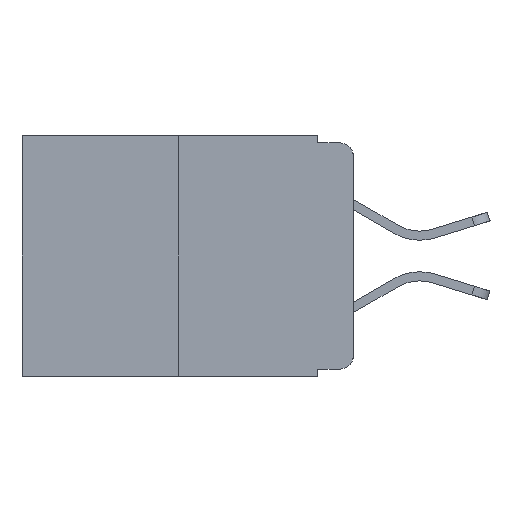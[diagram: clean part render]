
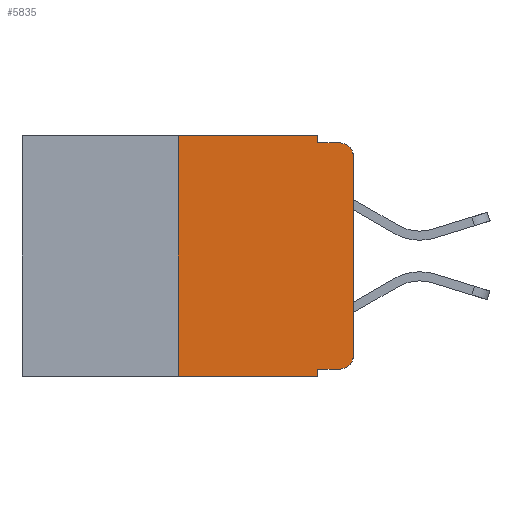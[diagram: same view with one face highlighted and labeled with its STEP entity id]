
A CAD part, left-side view. The second image highlights one B-rep face of the part: STEP entity #5835.
In plain terms, the highlighted planar face has unit normal (-1, 0, 0).
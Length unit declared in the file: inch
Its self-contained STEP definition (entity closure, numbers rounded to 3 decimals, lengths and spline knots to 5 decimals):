
#280 = DIRECTION ( 'NONE',  ( 0., 0., 1. ) ) ;
#578 = ORIENTED_EDGE ( 'NONE', *, *, #2444, .T. ) ;
#847 = DIRECTION ( 'NONE',  ( 0., 0., 1. ) ) ;
#1234 = CARTESIAN_POINT ( 'NONE',  ( 0., 0.25, 0. ) ) ;
#1261 = DIRECTION ( 'NONE',  ( 0., 0., -1. ) ) ;
#1451 = CARTESIAN_POINT ( 'NONE',  ( 0., 0., 0. ) ) ;
#1486 = DIRECTION ( 'NONE',  ( -1., 0., 0. ) ) ;
#1770 = EDGE_CURVE ( 'NONE', #8719, #7977, #2760, .T. ) ;
#1995 = VERTEX_POINT ( 'NONE', #3878 ) ;
#2293 = ORIENTED_EDGE ( 'NONE', *, *, #6491, .T. ) ;
#2437 = AXIS2_PLACEMENT_3D ( 'NONE', #7546, #1486, #8448 ) ;
#2444 = EDGE_CURVE ( 'NONE', #3549, #8719, #9752, .T. ) ;
#2611 = VECTOR ( 'NONE', #847, 39.37008 ) ;
#2659 = AXIS2_PLACEMENT_3D ( 'NONE', #9032, #11197, #12497 ) ;
#2755 = AXIS2_PLACEMENT_3D ( 'NONE', #6272, #4415, #4401 ) ;
#2760 = CIRCLE ( 'NONE', #2659, 0.02 ) ;
#2763 = CARTESIAN_POINT ( 'NONE',  ( 0., 0.473, 0. ) ) ;
#3030 = EDGE_LOOP ( 'NONE', ( #9432, #2293, #4907, #12263, #5556, #6881, #4759, #7770, #578, #8630 ) ) ;
#3115 = EDGE_CURVE ( 'NONE', #3549, #4345, #4777, .T. ) ;
#3549 = VERTEX_POINT ( 'NONE', #8162 ) ;
#3554 = VECTOR ( 'NONE', #8845, 39.37008 ) ;
#3674 = CARTESIAN_POINT ( 'NONE',  ( 0., 0., -0.313 ) ) ;
#3776 = EDGE_CURVE ( 'NONE', #5357, #1995, #7906, .T. ) ;
#3878 = CARTESIAN_POINT ( 'NONE',  ( 0., 0.25, 0. ) ) ;
#4345 = VERTEX_POINT ( 'NONE', #9505 ) ;
#4401 = DIRECTION ( 'NONE',  ( 0., 0., -1. ) ) ;
#4415 = DIRECTION ( 'NONE',  ( 1., 0., 0. ) ) ;
#4565 = DIRECTION ( 'NONE',  ( 0., -1., 0. ) ) ;
#4583 = CARTESIAN_POINT ( 'NONE',  ( 0., 0.051, -0.01 ) ) ;
#4759 = ORIENTED_EDGE ( 'NONE', *, *, #12245, .T. ) ;
#4777 = LINE ( 'NONE', #7247, #9591 ) ;
#4907 = ORIENTED_EDGE ( 'NONE', *, *, #5789, .F. ) ;
#5076 = EDGE_CURVE ( 'NONE', #10457, #11267, #9008, .T. ) ;
#5225 = PLANE ( 'NONE',  #2755 ) ;
#5357 = VERTEX_POINT ( 'NONE', #10521 ) ;
#5508 = CARTESIAN_POINT ( 'NONE',  ( 0., 0.051, -0.333 ) ) ;
#5556 = ORIENTED_EDGE ( 'NONE', *, *, #8328, .F. ) ;
#5789 = EDGE_CURVE ( 'NONE', #11267, #12074, #6635, .T. ) ;
#5825 = CARTESIAN_POINT ( 'NONE',  ( 0., 0.051, 0. ) ) ;
#5835 = ADVANCED_FACE ( 'NONE', ( #8256 ), #5225, .F. ) ;
#6272 = CARTESIAN_POINT ( 'NONE',  ( 0., 0.473, 0. ) ) ;
#6449 = CIRCLE ( 'NONE', #2437, 0.02 ) ;
#6491 = EDGE_CURVE ( 'NONE', #10526, #12074, #6449, .T. ) ;
#6549 = VECTOR ( 'NONE', #1261, 39.37008 ) ;
#6635 = LINE ( 'NONE', #4583, #8812 ) ;
#6881 = ORIENTED_EDGE ( 'NONE', *, *, #3776, .F. ) ;
#7247 = CARTESIAN_POINT ( 'NONE',  ( 0., 0.051, 0. ) ) ;
#7546 = CARTESIAN_POINT ( 'NONE',  ( 0., 0.02, -0.03 ) ) ;
#7645 = VECTOR ( 'NONE', #280, 39.37008 ) ;
#7770 = ORIENTED_EDGE ( 'NONE', *, *, #3115, .F. ) ;
#7778 = CARTESIAN_POINT ( 'NONE',  ( 0., 0.051, -0.01 ) ) ;
#7798 = EDGE_CURVE ( 'NONE', #7977, #10526, #7926, .T. ) ;
#7906 = LINE ( 'NONE', #1234, #2611 ) ;
#7926 = LINE ( 'NONE', #1451, #7645 ) ;
#7977 = VERTEX_POINT ( 'NONE', #3674 ) ;
#8162 = CARTESIAN_POINT ( 'NONE',  ( 0., 0.051, -0.333 ) ) ;
#8256 = FACE_OUTER_BOUND ( 'NONE', #3030, .T. ) ;
#8328 = EDGE_CURVE ( 'NONE', #1995, #10457, #11038, .T. ) ;
#8448 = DIRECTION ( 'NONE',  ( 0., 0., -1. ) ) ;
#8485 = LINE ( 'NONE', #10879, #10518 ) ;
#8630 = ORIENTED_EDGE ( 'NONE', *, *, #1770, .T. ) ;
#8719 = VERTEX_POINT ( 'NONE', #11844 ) ;
#8767 = CARTESIAN_POINT ( 'NONE',  ( 0., 0., -0.03 ) ) ;
#8807 = CARTESIAN_POINT ( 'NONE',  ( 0., 0.051, 0. ) ) ;
#8812 = VECTOR ( 'NONE', #4565, 39.37008 ) ;
#8845 = DIRECTION ( 'NONE',  ( 0., -1., 0. ) ) ;
#9008 = LINE ( 'NONE', #8807, #6549 ) ;
#9032 = CARTESIAN_POINT ( 'NONE',  ( 0., 0.02, -0.313 ) ) ;
#9432 = ORIENTED_EDGE ( 'NONE', *, *, #7798, .T. ) ;
#9505 = CARTESIAN_POINT ( 'NONE',  ( 0., 0.051, -0.343 ) ) ;
#9591 = VECTOR ( 'NONE', #12407, 39.37008 ) ;
#9752 = LINE ( 'NONE', #5508, #11745 ) ;
#10457 = VERTEX_POINT ( 'NONE', #5825 ) ;
#10506 = DIRECTION ( 'NONE',  ( 0., -1., 0. ) ) ;
#10518 = VECTOR ( 'NONE', #11746, 39.37008 ) ;
#10521 = CARTESIAN_POINT ( 'NONE',  ( 0., 0.25, -0.343 ) ) ;
#10526 = VERTEX_POINT ( 'NONE', #8767 ) ;
#10879 = CARTESIAN_POINT ( 'NONE',  ( 0., 0.473, -0.343 ) ) ;
#11038 = LINE ( 'NONE', #2763, #3554 ) ;
#11197 = DIRECTION ( 'NONE',  ( -1., 0., 0. ) ) ;
#11267 = VERTEX_POINT ( 'NONE', #7778 ) ;
#11745 = VECTOR ( 'NONE', #10506, 39.37008 ) ;
#11746 = DIRECTION ( 'NONE',  ( 0., -1., 0. ) ) ;
#11844 = CARTESIAN_POINT ( 'NONE',  ( 0., 0.02, -0.333 ) ) ;
#12074 = VERTEX_POINT ( 'NONE', #12400 ) ;
#12245 = EDGE_CURVE ( 'NONE', #5357, #4345, #8485, .T. ) ;
#12263 = ORIENTED_EDGE ( 'NONE', *, *, #5076, .F. ) ;
#12400 = CARTESIAN_POINT ( 'NONE',  ( 0., 0.02, -0.01 ) ) ;
#12407 = DIRECTION ( 'NONE',  ( 0., 0., -1. ) ) ;
#12497 = DIRECTION ( 'NONE',  ( 0., 0., -1. ) ) ;
